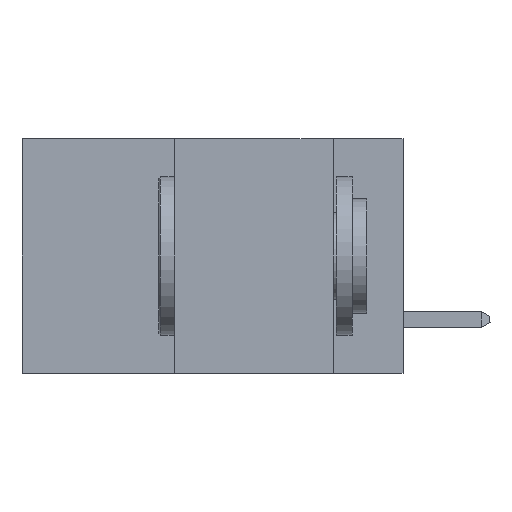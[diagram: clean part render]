
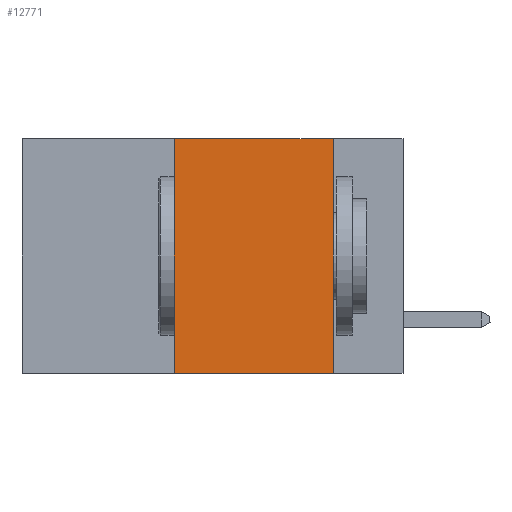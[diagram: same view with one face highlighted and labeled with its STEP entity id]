
A CAD part, left-side view. The second image highlights one B-rep face of the part: STEP entity #12771.
In plain terms, the highlighted planar face has unit normal (-1, 0, 0).
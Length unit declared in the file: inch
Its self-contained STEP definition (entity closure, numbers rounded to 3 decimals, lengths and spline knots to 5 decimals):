
#382 = VECTOR ( 'NONE', #4033, 39.37008 ) ;
#500 = VERTEX_POINT ( 'NONE', #3562 ) ;
#1485 = ORIENTED_EDGE ( 'NONE', *, *, #5615, .T. ) ;
#1497 = VERTEX_POINT ( 'NONE', #11362 ) ;
#1942 = CARTESIAN_POINT ( 'NONE',  ( 0., 0.36, 0. ) ) ;
#2357 = VERTEX_POINT ( 'NONE', #2859 ) ;
#2822 = CARTESIAN_POINT ( 'NONE',  ( 0., 0.11, 0. ) ) ;
#2859 = CARTESIAN_POINT ( 'NONE',  ( 0., 0.36, -0.37 ) ) ;
#3562 = CARTESIAN_POINT ( 'NONE',  ( 0., 0.36, 0. ) ) ;
#3641 = DIRECTION ( 'NONE',  ( 0., 0., -1. ) ) ;
#4033 = DIRECTION ( 'NONE',  ( 0., 0., -1. ) ) ;
#4242 = ORIENTED_EDGE ( 'NONE', *, *, #11462, .F. ) ;
#4810 = EDGE_CURVE ( 'NONE', #6937, #1497, #13325, .T. ) ;
#4853 = CARTESIAN_POINT ( 'NONE',  ( 0., 0.6, -0.37 ) ) ;
#5400 = DIRECTION ( 'NONE',  ( 0., 0., 1. ) ) ;
#5615 = EDGE_CURVE ( 'NONE', #2357, #1497, #9531, .T. ) ;
#6760 = CARTESIAN_POINT ( 'NONE',  ( 0., 0.11, 0. ) ) ;
#6797 = EDGE_LOOP ( 'NONE', ( #9947, #9182, #4242, #1485 ) ) ;
#6937 = VERTEX_POINT ( 'NONE', #6760 ) ;
#8273 = PLANE ( 'NONE',  #13906 ) ;
#8578 = FACE_OUTER_BOUND ( 'NONE', #6797, .T. ) ;
#8693 = EDGE_CURVE ( 'NONE', #500, #6937, #8727, .T. ) ;
#8727 = LINE ( 'NONE', #8894, #8902 ) ;
#8894 = CARTESIAN_POINT ( 'NONE',  ( 0., 0.6, 0. ) ) ;
#8902 = VECTOR ( 'NONE', #11210, 39.37008 ) ;
#9182 = ORIENTED_EDGE ( 'NONE', *, *, #8693, .F. ) ;
#9531 = LINE ( 'NONE', #4853, #10066 ) ;
#9947 = ORIENTED_EDGE ( 'NONE', *, *, #4810, .F. ) ;
#10066 = VECTOR ( 'NONE', #10736, 39.37008 ) ;
#10736 = DIRECTION ( 'NONE',  ( 0., -1., 0. ) ) ;
#11210 = DIRECTION ( 'NONE',  ( 0., -1., 0. ) ) ;
#11362 = CARTESIAN_POINT ( 'NONE',  ( 0., 0.11, -0.37 ) ) ;
#11462 = EDGE_CURVE ( 'NONE', #2357, #500, #13146, .T. ) ;
#11765 = CARTESIAN_POINT ( 'NONE',  ( 0., 0.6, 0. ) ) ;
#11815 = DIRECTION ( 'NONE',  ( 1., 0., 0. ) ) ;
#12771 = ADVANCED_FACE ( 'NONE', ( #8578 ), #8273, .F. ) ;
#13146 = LINE ( 'NONE', #1942, #15129 ) ;
#13325 = LINE ( 'NONE', #2822, #382 ) ;
#13906 = AXIS2_PLACEMENT_3D ( 'NONE', #11765, #11815, #3641 ) ;
#15129 = VECTOR ( 'NONE', #5400, 39.37008 ) ;
